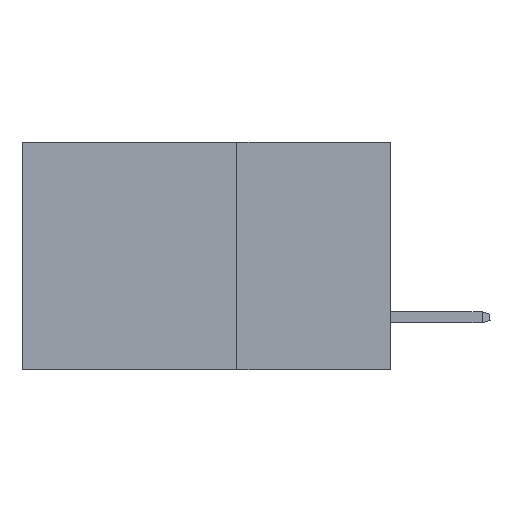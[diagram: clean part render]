
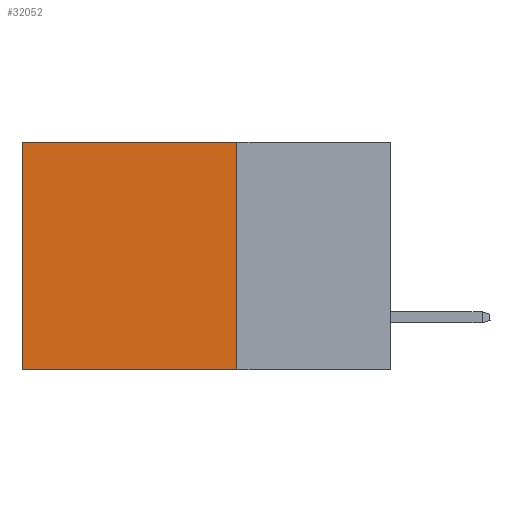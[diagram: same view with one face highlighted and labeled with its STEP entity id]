
A CAD part, left-side view. The second image highlights one B-rep face of the part: STEP entity #32052.
In plain terms, the highlighted planar face has unit normal (-1, 0, 0).
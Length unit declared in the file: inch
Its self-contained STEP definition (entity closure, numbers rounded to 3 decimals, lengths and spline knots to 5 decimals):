
#1383 = CARTESIAN_POINT ( 'NONE',  ( 0.2875, 0.25, 0. ) ) ;
#3072 = LINE ( 'NONE', #11454, #32272 ) ;
#3808 = VERTEX_POINT ( 'NONE', #20992 ) ;
#3933 = LINE ( 'NONE', #30105, #33134 ) ;
#4435 = VECTOR ( 'NONE', #12988, 39.37008 ) ;
#5446 = DIRECTION ( 'NONE',  ( 0., 1., 0. ) ) ;
#6656 = LINE ( 'NONE', #12482, #4435 ) ;
#6972 = CARTESIAN_POINT ( 'NONE',  ( 0.2875, 0.6, 0. ) ) ;
#7081 = FACE_OUTER_BOUND ( 'NONE', #30098, .T. ) ;
#8031 = DIRECTION ( 'NONE',  ( 0., 0., -1. ) ) ;
#8415 = DIRECTION ( 'NONE',  ( 0., 1., 0. ) ) ;
#11454 = CARTESIAN_POINT ( 'NONE',  ( 0.2875, 0.25, -0.37 ) ) ;
#12482 = CARTESIAN_POINT ( 'NONE',  ( 0.2875, 0.6, 0. ) ) ;
#12988 = DIRECTION ( 'NONE',  ( 0., 0., -1. ) ) ;
#13848 = CARTESIAN_POINT ( 'NONE',  ( 0.2875, 0.25, -0.37 ) ) ;
#15302 = EDGE_CURVE ( 'NONE', #23507, #3808, #3072, .T. ) ;
#17735 = LINE ( 'NONE', #1383, #31494 ) ;
#18974 = CARTESIAN_POINT ( 'NONE',  ( 0.2875, 0.25, 0. ) ) ;
#18984 = VERTEX_POINT ( 'NONE', #6972 ) ;
#20992 = CARTESIAN_POINT ( 'NONE',  ( 0.2875, 0.6, -0.37 ) ) ;
#21355 = ORIENTED_EDGE ( 'NONE', *, *, #34519, .F. ) ;
#22083 = DIRECTION ( 'NONE',  ( 1., 0., 0. ) ) ;
#22270 = EDGE_CURVE ( 'NONE', #33898, #18984, #3933, .T. ) ;
#23507 = VERTEX_POINT ( 'NONE', #13848 ) ;
#24689 = CARTESIAN_POINT ( 'NONE',  ( 0.2875, 0.25, 0. ) ) ;
#24942 = DIRECTION ( 'NONE',  ( 0., 0., -1. ) ) ;
#27401 = EDGE_CURVE ( 'NONE', #18984, #3808, #6656, .T. ) ;
#28536 = AXIS2_PLACEMENT_3D ( 'NONE', #18974, #22083, #24942 ) ;
#28676 = ORIENTED_EDGE ( 'NONE', *, *, #15302, .F. ) ;
#29277 = ORIENTED_EDGE ( 'NONE', *, *, #27401, .T. ) ;
#30098 = EDGE_LOOP ( 'NONE', ( #29277, #28676, #21355, #32112 ) ) ;
#30105 = CARTESIAN_POINT ( 'NONE',  ( 0.2875, 0.25, 0. ) ) ;
#31494 = VECTOR ( 'NONE', #8031, 39.37008 ) ;
#32052 = ADVANCED_FACE ( 'NONE', ( #7081 ), #32952, .F. ) ;
#32112 = ORIENTED_EDGE ( 'NONE', *, *, #22270, .T. ) ;
#32272 = VECTOR ( 'NONE', #5446, 39.37008 ) ;
#32952 = PLANE ( 'NONE',  #28536 ) ;
#33134 = VECTOR ( 'NONE', #8415, 39.37008 ) ;
#33898 = VERTEX_POINT ( 'NONE', #24689 ) ;
#34519 = EDGE_CURVE ( 'NONE', #33898, #23507, #17735, .T. ) ;
